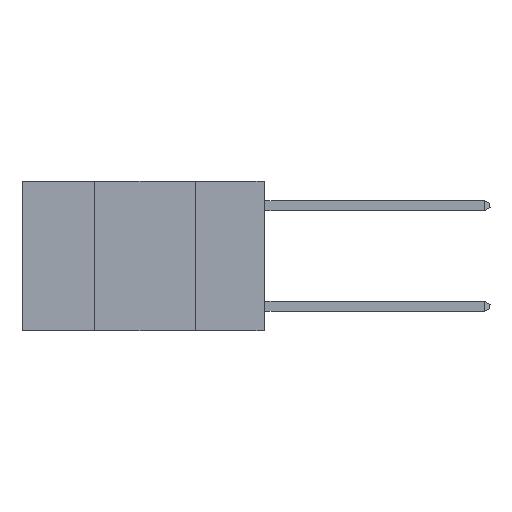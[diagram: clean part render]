
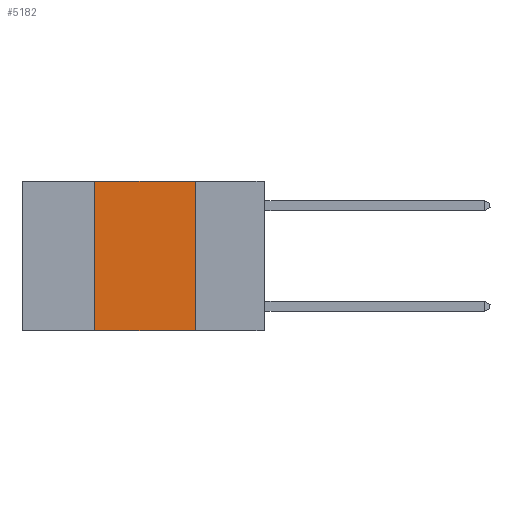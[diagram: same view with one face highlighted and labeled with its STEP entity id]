
A CAD part, left-side view. The second image highlights one B-rep face of the part: STEP entity #5182.
In plain terms, the highlighted planar face has unit normal (-1, 0, 0).
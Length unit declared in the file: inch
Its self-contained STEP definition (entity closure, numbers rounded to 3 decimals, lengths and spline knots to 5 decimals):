
#18 = CARTESIAN_POINT ( 'NONE',  ( 0., 0.17, 0. ) ) ;
#1476 = ORIENTED_EDGE ( 'NONE', *, *, #21140, .F. ) ;
#1694 = FACE_OUTER_BOUND ( 'NONE', #3043, .T. ) ;
#3043 = EDGE_LOOP ( 'NONE', ( #4392, #3496, #1476, #15996 ) ) ;
#3496 = ORIENTED_EDGE ( 'NONE', *, *, #9338, .F. ) ;
#3555 = DIRECTION ( 'NONE',  ( 0., 0., -1. ) ) ;
#3771 = VECTOR ( 'NONE', #9956, 39.37008 ) ;
#4392 = ORIENTED_EDGE ( 'NONE', *, *, #9187, .F. ) ;
#4590 = CARTESIAN_POINT ( 'NONE',  ( 0., 0.17, 0. ) ) ;
#5182 = ADVANCED_FACE ( 'NONE', ( #1694 ), #21367, .F. ) ;
#6803 = CARTESIAN_POINT ( 'NONE',  ( 0., 0.42, 0. ) ) ;
#6869 = AXIS2_PLACEMENT_3D ( 'NONE', #14378, #16810, #3555 ) ;
#8658 = VERTEX_POINT ( 'NONE', #6803 ) ;
#9187 = EDGE_CURVE ( 'NONE', #15726, #13847, #19669, .T. ) ;
#9338 = EDGE_CURVE ( 'NONE', #8658, #15726, #16243, .T. ) ;
#9956 = DIRECTION ( 'NONE',  ( 0., -1., 0. ) ) ;
#10998 = DIRECTION ( 'NONE',  ( 0., 0., -1. ) ) ;
#11726 = EDGE_CURVE ( 'NONE', #26712, #13847, #19674, .T. ) ;
#13051 = CARTESIAN_POINT ( 'NONE',  ( 0., 0.42, -0.37 ) ) ;
#13279 = CARTESIAN_POINT ( 'NONE',  ( 0., 0.42, 0. ) ) ;
#13847 = VERTEX_POINT ( 'NONE', #16848 ) ;
#14378 = CARTESIAN_POINT ( 'NONE',  ( 0., 0.6, 0. ) ) ;
#15726 = VERTEX_POINT ( 'NONE', #18 ) ;
#15996 = ORIENTED_EDGE ( 'NONE', *, *, #11726, .T. ) ;
#16243 = LINE ( 'NONE', #18229, #3771 ) ;
#16507 = VECTOR ( 'NONE', #10998, 39.37008 ) ;
#16810 = DIRECTION ( 'NONE',  ( 1., 0., 0. ) ) ;
#16848 = CARTESIAN_POINT ( 'NONE',  ( 0., 0.17, -0.37 ) ) ;
#17589 = VECTOR ( 'NONE', #26130, 39.37008 ) ;
#18229 = CARTESIAN_POINT ( 'NONE',  ( 0., 0.6, 0. ) ) ;
#19669 = LINE ( 'NONE', #4590, #16507 ) ;
#19674 = LINE ( 'NONE', #25674, #24340 ) ;
#21140 = EDGE_CURVE ( 'NONE', #26712, #8658, #22245, .T. ) ;
#21367 = PLANE ( 'NONE',  #6869 ) ;
#22245 = LINE ( 'NONE', #13279, #17589 ) ;
#24340 = VECTOR ( 'NONE', #25824, 39.37008 ) ;
#25674 = CARTESIAN_POINT ( 'NONE',  ( 0., 0.6, -0.37 ) ) ;
#25824 = DIRECTION ( 'NONE',  ( 0., -1., 0. ) ) ;
#26130 = DIRECTION ( 'NONE',  ( 0., 0., 1. ) ) ;
#26712 = VERTEX_POINT ( 'NONE', #13051 ) ;
